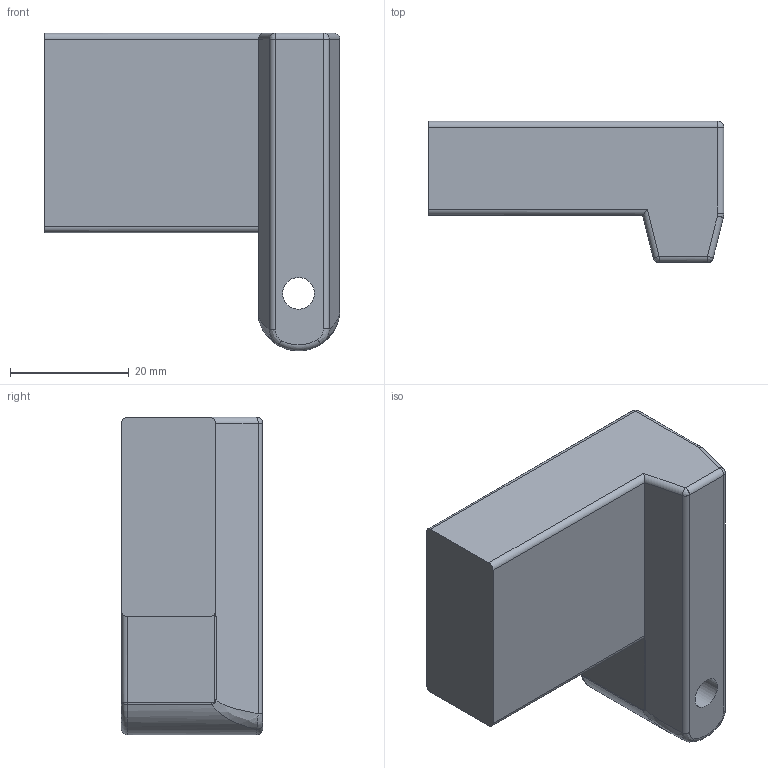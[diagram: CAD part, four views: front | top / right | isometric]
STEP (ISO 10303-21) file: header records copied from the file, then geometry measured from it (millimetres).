
FILE_DESCRIPTION (( 'STEP AP203' ), '1' );
FILE_NAME ('WTF-9_stock_lock.STEP', '2020-05-09T10:06:49', ( '' ), ( '' ), 'SwSTEP 2.0', 'SolidWorks 2016', '' );
FILE_SCHEMA (( 'CONFIG_CONTROL_DESIGN' ));
Length unit declared in the file: millimetre
Products named in the file (2): WTF-9_stock_lock; WTF9 V1 FINAL_2
Assembly tree (1 placements, depth 2):
  WTF-9_stock_lock
    WTF9 V1 FINAL_2
Bounding box: 49.75 x 23.76 x 53.45 mm (x, y, z)
Volume: 34681.6 mm3; surface area: 8041.6 mm2
Topology: 1 solids, 1 shells, 43 faces, 103 edges, 59 vertices
Faces by surface type: cylinder 17, plane 13, bspline 7, torus 3, sphere 2, cone 1
Full cylindrical faces by diameter (mm): 5.346 x1
Entity records: 1587 total; most frequent: CARTESIAN_POINT 483, ORIENTED_EDGE 196, DIRECTION 179, EDGE_CURVE 98, AXIS2_PLACEMENT_3D 68, VERTEX_POINT 59, EDGE_LOOP 47, FACE_OUTER_BOUND 44
